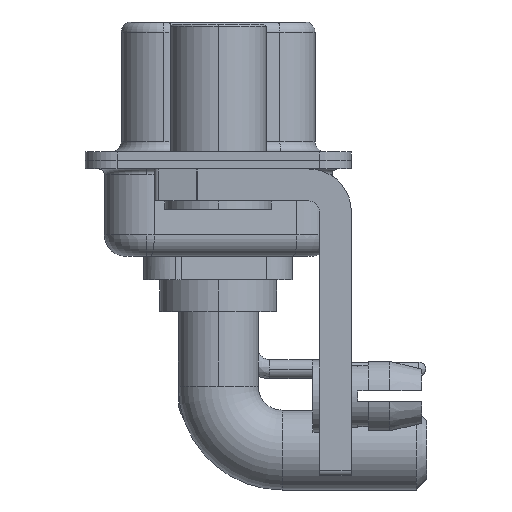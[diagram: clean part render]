
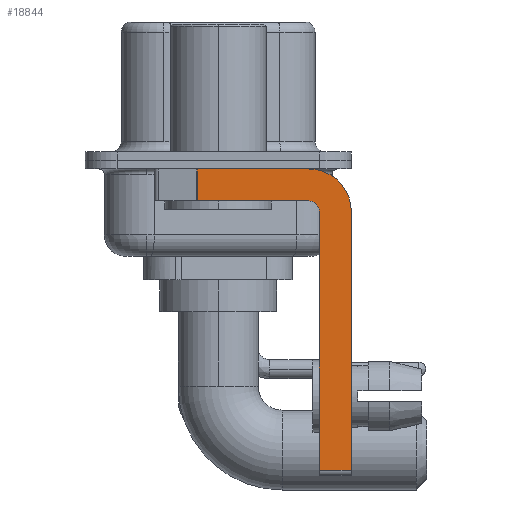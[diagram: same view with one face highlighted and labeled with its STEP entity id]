
A CAD part, left-side view. The second image highlights one B-rep face of the part: STEP entity #18844.
In plain terms, the highlighted planar face has unit normal (-1, 0, 0).
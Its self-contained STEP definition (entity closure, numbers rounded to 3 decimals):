
#393 = CARTESIAN_POINT ( 'NONE',  ( -2.9, -4.25, -2.4 ) ) ;
#411 = PLANE ( 'NONE',  #14639 ) ;
#883 = VECTOR ( 'NONE', #24761, 1000. ) ;
#925 = CARTESIAN_POINT ( 'NONE',  ( -2.9, 0.978, -1.9 ) ) ;
#1020 = EDGE_CURVE ( 'NONE', #16746, #20161, #25946, .T. ) ;
#1708 = LINE ( 'NONE', #18103, #14281 ) ;
#1989 = VERTEX_POINT ( 'NONE', #3546 ) ;
#2812 = CARTESIAN_POINT ( 'NONE',  ( -2.9, -4.75, -14.55 ) ) ;
#2966 = AXIS2_PLACEMENT_3D ( 'NONE', #7729, #11758, #5957 ) ;
#3546 = CARTESIAN_POINT ( 'NONE',  ( -2.9, -4.75, -2.4 ) ) ;
#4183 = CIRCLE ( 'NONE', #14479, 0.5 ) ;
#4983 = DIRECTION ( 'NONE',  ( 0., 0., -1. ) ) ;
#5194 = LINE ( 'NONE', #7071, #18800 ) ;
#5251 = ORIENTED_EDGE ( 'NONE', *, *, #1020, .T. ) ;
#5587 = EDGE_CURVE ( 'NONE', #20205, #1989, #1708, .T. ) ;
#5589 = ORIENTED_EDGE ( 'NONE', *, *, #20728, .F. ) ;
#5911 = EDGE_CURVE ( 'NONE', #6674, #6707, #25595, .T. ) ;
#5957 = DIRECTION ( 'NONE',  ( 0., 0., -1. ) ) ;
#6467 = CARTESIAN_POINT ( 'NONE',  ( -2.9, -6.25, -14.55 ) ) ;
#6674 = VERTEX_POINT ( 'NONE', #24232 ) ;
#6707 = VERTEX_POINT ( 'NONE', #6467 ) ;
#7071 = CARTESIAN_POINT ( 'NONE',  ( -2.9, -4.25, -1.9 ) ) ;
#7327 = CARTESIAN_POINT ( 'NONE',  ( -2.9, -4.25, -1.9 ) ) ;
#7729 = CARTESIAN_POINT ( 'NONE',  ( -2.9, -4.25, -2.4 ) ) ;
#7843 = ORIENTED_EDGE ( 'NONE', *, *, #13842, .F. ) ;
#8489 = EDGE_LOOP ( 'NONE', ( #22803, #5251, #5589, #7843, #8618, #8539, #10781, #21943 ) ) ;
#8539 = ORIENTED_EDGE ( 'NONE', *, *, #18623, .T. ) ;
#8618 = ORIENTED_EDGE ( 'NONE', *, *, #5587, .F. ) ;
#9807 = VECTOR ( 'NONE', #22342, 1000. ) ;
#10269 = CIRCLE ( 'NONE', #2966, 2. ) ;
#10781 = ORIENTED_EDGE ( 'NONE', *, *, #5911, .F. ) ;
#11758 = DIRECTION ( 'NONE',  ( 1., 0., 0. ) ) ;
#13212 = EDGE_CURVE ( 'NONE', #16746, #20340, #16295, .T. ) ;
#13842 = EDGE_CURVE ( 'NONE', #1989, #15156, #4183, .T. ) ;
#14281 = VECTOR ( 'NONE', #26314, 1000. ) ;
#14479 = AXIS2_PLACEMENT_3D ( 'NONE', #393, #18563, #22471 ) ;
#14639 = AXIS2_PLACEMENT_3D ( 'NONE', #23123, #14810, #4983 ) ;
#14787 = CARTESIAN_POINT ( 'NONE',  ( -2.9, 0.978, -1.9 ) ) ;
#14810 = DIRECTION ( 'NONE',  ( 1., 0., 0. ) ) ;
#15156 = VERTEX_POINT ( 'NONE', #7327 ) ;
#16164 = LINE ( 'NONE', #20727, #883 ) ;
#16295 = LINE ( 'NONE', #23863, #9807 ) ;
#16746 = VERTEX_POINT ( 'NONE', #24916 ) ;
#16873 = CARTESIAN_POINT ( 'NONE',  ( -2.9, -6.25, -2.4 ) ) ;
#17392 = DIRECTION ( 'NONE',  ( 0., 0., -1. ) ) ;
#17734 = DIRECTION ( 'NONE',  ( 0., 0., -1. ) ) ;
#18103 = CARTESIAN_POINT ( 'NONE',  ( -2.9, -4.75, -14.8 ) ) ;
#18563 = DIRECTION ( 'NONE',  ( -1., 0., 0. ) ) ;
#18623 = EDGE_CURVE ( 'NONE', #20205, #6707, #16164, .T. ) ;
#18800 = VECTOR ( 'NONE', #23596, 1000. ) ;
#18844 = ADVANCED_FACE ( 'NONE', ( #22870 ), #411, .F. ) ;
#19388 = VECTOR ( 'NONE', #17392, 1000. ) ;
#20161 = VERTEX_POINT ( 'NONE', #14787 ) ;
#20205 = VERTEX_POINT ( 'NONE', #2812 ) ;
#20340 = VERTEX_POINT ( 'NONE', #25797 ) ;
#20727 = CARTESIAN_POINT ( 'NONE',  ( -2.9, -4.25, -14.55 ) ) ;
#20728 = EDGE_CURVE ( 'NONE', #15156, #20161, #5194, .T. ) ;
#21262 = EDGE_CURVE ( 'NONE', #20340, #6674, #10269, .T. ) ;
#21943 = ORIENTED_EDGE ( 'NONE', *, *, #21262, .F. ) ;
#22051 = VECTOR ( 'NONE', #17734, 1000. ) ;
#22342 = DIRECTION ( 'NONE',  ( 0., -1., 0. ) ) ;
#22471 = DIRECTION ( 'NONE',  ( 0., 0., 1. ) ) ;
#22803 = ORIENTED_EDGE ( 'NONE', *, *, #13212, .F. ) ;
#22870 = FACE_OUTER_BOUND ( 'NONE', #8489, .T. ) ;
#23123 = CARTESIAN_POINT ( 'NONE',  ( -2.9, -4.25, -2.4 ) ) ;
#23596 = DIRECTION ( 'NONE',  ( 0., 1., 0. ) ) ;
#23863 = CARTESIAN_POINT ( 'NONE',  ( -2.9, 3., -0.4 ) ) ;
#24232 = CARTESIAN_POINT ( 'NONE',  ( -2.9, -6.25, -2.4 ) ) ;
#24761 = DIRECTION ( 'NONE',  ( 0., -1., 0. ) ) ;
#24916 = CARTESIAN_POINT ( 'NONE',  ( -2.9, 0.978, -0.4 ) ) ;
#25595 = LINE ( 'NONE', #16873, #19388 ) ;
#25797 = CARTESIAN_POINT ( 'NONE',  ( -2.9, -4.25, -0.4 ) ) ;
#25946 = LINE ( 'NONE', #925, #22051 ) ;
#26314 = DIRECTION ( 'NONE',  ( 0., 0., 1. ) ) ;
